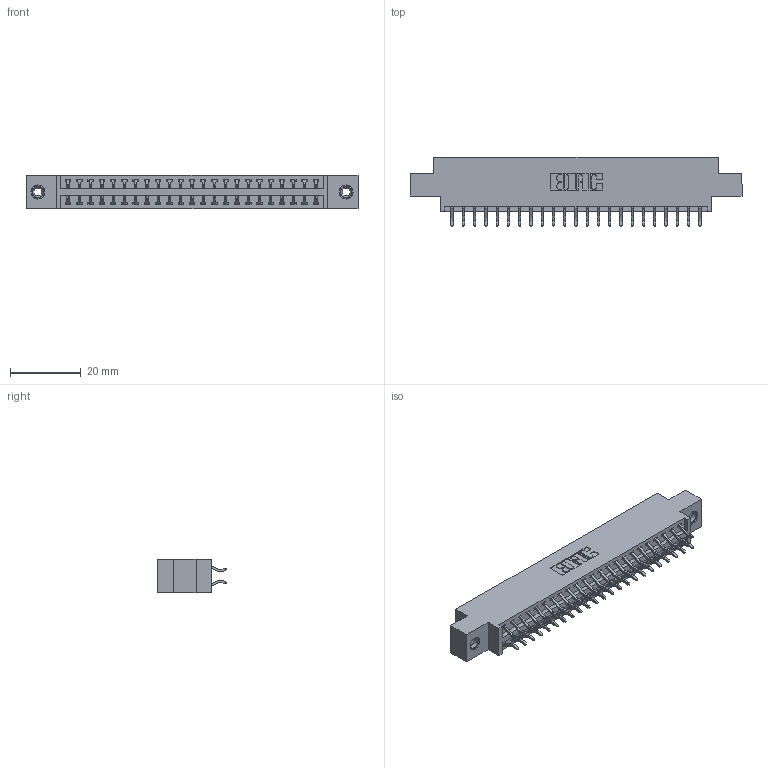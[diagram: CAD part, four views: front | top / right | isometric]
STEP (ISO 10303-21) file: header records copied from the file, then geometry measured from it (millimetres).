
FILE_DESCRIPTION (( 'STEP AP203' ), '1' );
FILE_NAME ('346-046-556-808.STEP', '2022-05-20T20:24:32', ( '' ), ( '' ), 'SwSTEP 2.0', 'SolidWorks 2020', '' );
FILE_SCHEMA (( 'CONFIG_CONTROL_DESIGN' ));
Length unit declared in the file: inch
Products named in the file (4): 345-250-001_345-250-003-102; 345-292-001_556 Tail; 346 Part_0.170 Offset - 0.156 Dia-TI; 346-046-556-808
Assembly tree (49 placements, depth 2):
  346-046-556-808
    346 Part_0.170 Offset - 0.156 Dia-TI
    345-292-001_556 Tail  x46
    345-250-001_345-250-003-102  x2
Bounding box: 93.6 x 19.57 x 9.4 mm (x, y, z)
Volume: 8816.5 mm3; surface area: 11977.2 mm2
Topology: 49 solids, 49 shells, 2854 faces, 8435 edges, 5554 vertices
Faces by surface type: plane 1906, cylinder 932, cone 12, torus 4
Entity records: 19106 total; most frequent: CARTESIAN_POINT 3175, ORIENTED_EDGE 3090, DIRECTION 2863, EDGE_CURVE 1545, VECTOR 1293, LINE 1293, VERTEX_POINT 1024, AXIS2_PLACEMENT_3D 785
